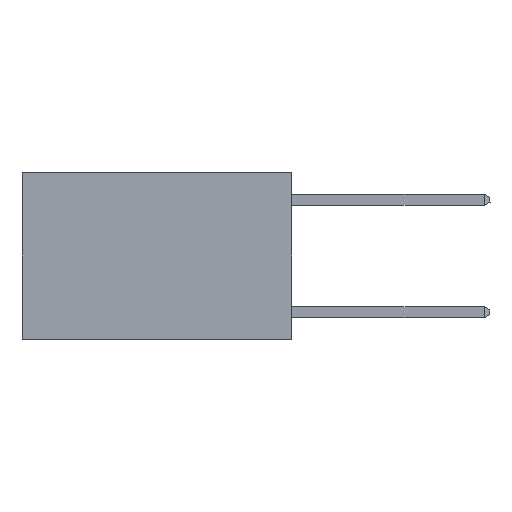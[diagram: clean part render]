
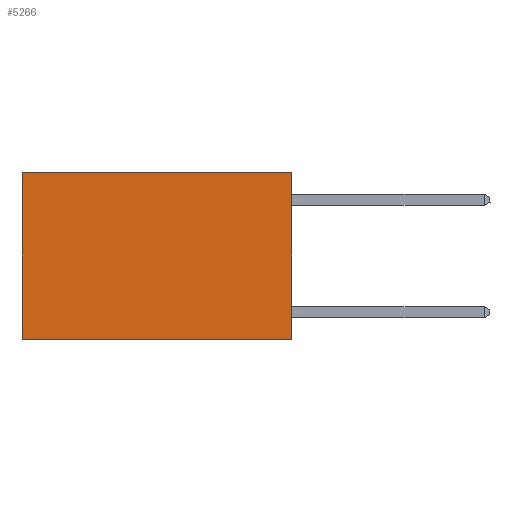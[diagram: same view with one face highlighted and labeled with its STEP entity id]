
A CAD part, left-side view. The second image highlights one B-rep face of the part: STEP entity #5266.
In plain terms, the highlighted planar face has unit normal (-1, 0, 0).
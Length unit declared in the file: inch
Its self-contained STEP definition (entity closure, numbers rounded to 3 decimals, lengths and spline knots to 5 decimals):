
#357 = DIRECTION ( 'NONE',  ( 0., 0., -1. ) ) ;
#628 = EDGE_CURVE ( 'NONE', #2770, #6374, #646, .T. ) ;
#646 = LINE ( 'NONE', #650, #6188 ) ;
#650 = CARTESIAN_POINT ( 'NONE',  ( 0.2625, 0., 0. ) ) ;
#915 = DIRECTION ( 'NONE',  ( 0., 1., 0. ) ) ;
#1178 = VECTOR ( 'NONE', #915, 39.37008 ) ;
#1348 = CARTESIAN_POINT ( 'NONE',  ( 0.2625, 0., 0. ) ) ;
#1432 = FACE_OUTER_BOUND ( 'NONE', #8020, .T. ) ;
#1484 = DIRECTION ( 'NONE',  ( 0., 0., -1. ) ) ;
#1580 = PLANE ( 'NONE',  #3216 ) ;
#2054 = LINE ( 'NONE', #5654, #1178 ) ;
#2063 = EDGE_CURVE ( 'NONE', #2770, #6774, #6482, .T. ) ;
#2190 = LINE ( 'NONE', #2417, #5452 ) ;
#2417 = CARTESIAN_POINT ( 'NONE',  ( 0.2625, 0.6, 0. ) ) ;
#2770 = VERTEX_POINT ( 'NONE', #5665 ) ;
#3000 = DIRECTION ( 'NONE',  ( 0., 0., -1. ) ) ;
#3216 = AXIS2_PLACEMENT_3D ( 'NONE', #7848, #3615, #3000 ) ;
#3615 = DIRECTION ( 'NONE',  ( 1., 0., 0. ) ) ;
#3777 = VECTOR ( 'NONE', #4137, 39.37008 ) ;
#3787 = CARTESIAN_POINT ( 'NONE',  ( 0.2625, 0., -0.37 ) ) ;
#3891 = CARTESIAN_POINT ( 'NONE',  ( 0.2625, 0.6, -0.37 ) ) ;
#4137 = DIRECTION ( 'NONE',  ( 0., 1., 0. ) ) ;
#4667 = EDGE_CURVE ( 'NONE', #6774, #7767, #2190, .T. ) ;
#5062 = ORIENTED_EDGE ( 'NONE', *, *, #2063, .T. ) ;
#5266 = ADVANCED_FACE ( 'NONE', ( #1432 ), #1580, .F. ) ;
#5452 = VECTOR ( 'NONE', #357, 39.37008 ) ;
#5519 = ORIENTED_EDGE ( 'NONE', *, *, #4667, .T. ) ;
#5654 = CARTESIAN_POINT ( 'NONE',  ( 0.2625, 0., -0.37 ) ) ;
#5665 = CARTESIAN_POINT ( 'NONE',  ( 0.2625, 0., 0. ) ) ;
#5982 = ORIENTED_EDGE ( 'NONE', *, *, #628, .F. ) ;
#6188 = VECTOR ( 'NONE', #1484, 39.37008 ) ;
#6374 = VERTEX_POINT ( 'NONE', #3787 ) ;
#6482 = LINE ( 'NONE', #1348, #3777 ) ;
#6628 = EDGE_CURVE ( 'NONE', #6374, #7767, #2054, .T. ) ;
#6774 = VERTEX_POINT ( 'NONE', #8950 ) ;
#7680 = ORIENTED_EDGE ( 'NONE', *, *, #6628, .F. ) ;
#7767 = VERTEX_POINT ( 'NONE', #3891 ) ;
#7848 = CARTESIAN_POINT ( 'NONE',  ( 0.2625, 0., 0. ) ) ;
#8020 = EDGE_LOOP ( 'NONE', ( #5519, #7680, #5982, #5062 ) ) ;
#8950 = CARTESIAN_POINT ( 'NONE',  ( 0.2625, 0.6, 0. ) ) ;
